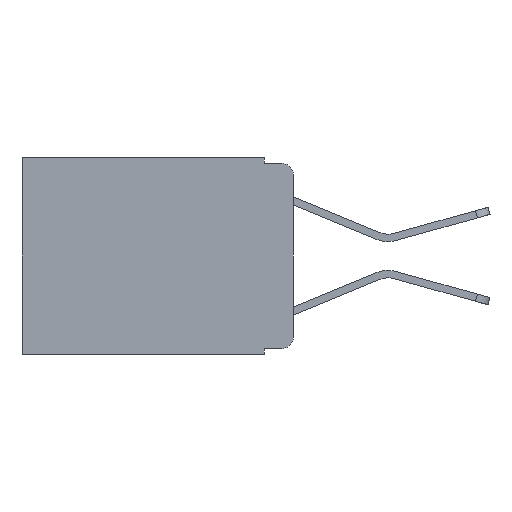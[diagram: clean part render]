
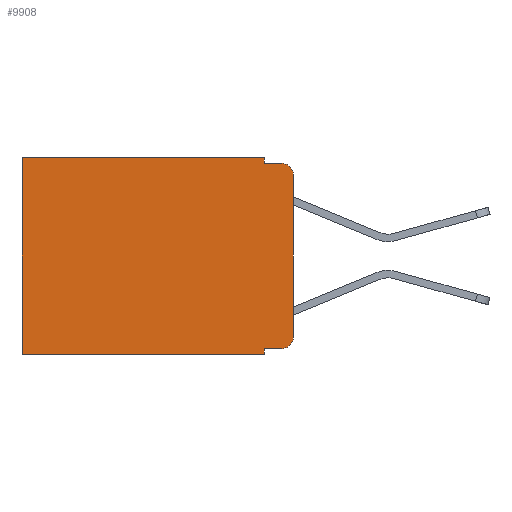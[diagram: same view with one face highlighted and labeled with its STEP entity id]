
A CAD part, left-side view. The second image highlights one B-rep face of the part: STEP entity #9908.
In plain terms, the highlighted planar face has unit normal (-1, 0, 0).
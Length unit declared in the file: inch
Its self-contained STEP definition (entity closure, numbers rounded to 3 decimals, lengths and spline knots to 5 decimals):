
#214 = LINE ( 'NONE', #10549, #2378 ) ;
#764 = ORIENTED_EDGE ( 'NONE', *, *, #7181, .F. ) ;
#981 = ORIENTED_EDGE ( 'NONE', *, *, #8253, .T. ) ;
#994 = ORIENTED_EDGE ( 'NONE', *, *, #7713, .F. ) ;
#1127 = LINE ( 'NONE', #5479, #7815 ) ;
#1152 = DIRECTION ( 'NONE',  ( 1., 0., 0. ) ) ;
#1216 = VECTOR ( 'NONE', #4176, 39.37008 ) ;
#1220 = LINE ( 'NONE', #7101, #10017 ) ;
#1238 = ORIENTED_EDGE ( 'NONE', *, *, #6210, .F. ) ;
#1242 = ORIENTED_EDGE ( 'NONE', *, *, #3553, .F. ) ;
#1414 = ORIENTED_EDGE ( 'NONE', *, *, #7021, .T. ) ;
#1642 = ORIENTED_EDGE ( 'NONE', *, *, #5609, .T. ) ;
#1786 = DIRECTION ( 'NONE',  ( 0., 1., 0. ) ) ;
#1809 = CARTESIAN_POINT ( 'NONE',  ( 0.298, 0.051, -0.01 ) ) ;
#1814 = ORIENTED_EDGE ( 'NONE', *, *, #4394, .T. ) ;
#2066 = DIRECTION ( 'NONE',  ( -1., 0., 0. ) ) ;
#2099 = ORIENTED_EDGE ( 'NONE', *, *, #6758, .T. ) ;
#2120 = CARTESIAN_POINT ( 'NONE',  ( 0.298, 0.02, -0.313 ) ) ;
#2212 = DIRECTION ( 'NONE',  ( 0., 1., 0. ) ) ;
#2268 = ORIENTED_EDGE ( 'NONE', *, *, #2658, .F. ) ;
#2378 = VECTOR ( 'NONE', #2212, 39.37008 ) ;
#2413 = CARTESIAN_POINT ( 'NONE',  ( 0.298, 0., 0. ) ) ;
#2505 = AXIS2_PLACEMENT_3D ( 'NONE', #2120, #9318, #7518 ) ;
#2546 = LINE ( 'NONE', #9538, #7183 ) ;
#2658 = EDGE_CURVE ( 'NONE', #5961, #5140, #1127, .T. ) ;
#2748 = FACE_OUTER_BOUND ( 'NONE', #7191, .T. ) ;
#3095 = CIRCLE ( 'NONE', #2505, 0.02 ) ;
#3159 = DIRECTION ( 'NONE',  ( 0., -1., 0. ) ) ;
#3375 = LINE ( 'NONE', #2413, #1216 ) ;
#3553 = EDGE_CURVE ( 'NONE', #5140, #5456, #2546, .T. ) ;
#4016 = CARTESIAN_POINT ( 'NONE',  ( 0.298, 0.051, -0.01 ) ) ;
#4176 = DIRECTION ( 'NONE',  ( 0., 0., -1. ) ) ;
#4394 = EDGE_CURVE ( 'NONE', #5961, #10137, #1220, .T. ) ;
#4582 = CARTESIAN_POINT ( 'NONE',  ( 0.298, 0.02, -0.01 ) ) ;
#4684 = VECTOR ( 'NONE', #5837, 39.37008 ) ;
#4763 = VERTEX_POINT ( 'NONE', #8011 ) ;
#4827 = CARTESIAN_POINT ( 'NONE',  ( 0.298, 0.051, 0. ) ) ;
#4924 = VERTEX_POINT ( 'NONE', #4582 ) ;
#5134 = LINE ( 'NONE', #4016, #7397 ) ;
#5140 = VERTEX_POINT ( 'NONE', #10711 ) ;
#5454 = DIRECTION ( 'NONE',  ( 0., 0., -1. ) ) ;
#5456 = VERTEX_POINT ( 'NONE', #10879 ) ;
#5479 = CARTESIAN_POINT ( 'NONE',  ( 0.298, 0.051, 0. ) ) ;
#5492 = VERTEX_POINT ( 'NONE', #10755 ) ;
#5609 = EDGE_CURVE ( 'NONE', #9261, #5456, #8527, .T. ) ;
#5837 = DIRECTION ( 'NONE',  ( 0., 0., -1. ) ) ;
#5961 = VERTEX_POINT ( 'NONE', #8649 ) ;
#6088 = VECTOR ( 'NONE', #9145, 39.37008 ) ;
#6210 = EDGE_CURVE ( 'NONE', #4763, #9373, #7249, .T. ) ;
#6714 = AXIS2_PLACEMENT_3D ( 'NONE', #7296, #2066, #8105 ) ;
#6758 = EDGE_CURVE ( 'NONE', #10137, #5492, #3095, .T. ) ;
#6839 = CARTESIAN_POINT ( 'NONE',  ( 0.298, 0.02, -0.333 ) ) ;
#7021 = EDGE_CURVE ( 'NONE', #4763, #9261, #214, .T. ) ;
#7101 = CARTESIAN_POINT ( 'NONE',  ( 0.298, 0.051, -0.333 ) ) ;
#7181 = EDGE_CURVE ( 'NONE', #7731, #5492, #3375, .T. ) ;
#7183 = VECTOR ( 'NONE', #1786, 39.37008 ) ;
#7191 = EDGE_LOOP ( 'NONE', ( #764, #981, #994, #1238, #1414, #1642, #1242, #2268, #1814, #2099 ) ) ;
#7249 = LINE ( 'NONE', #4827, #4684 ) ;
#7275 = CARTESIAN_POINT ( 'NONE',  ( 0.298, 0., 0. ) ) ;
#7296 = CARTESIAN_POINT ( 'NONE',  ( 0.298, 0.02, -0.03 ) ) ;
#7307 = DIRECTION ( 'NONE',  ( 0., 0., -1. ) ) ;
#7397 = VECTOR ( 'NONE', #9065, 39.37008 ) ;
#7518 = DIRECTION ( 'NONE',  ( 0., 0., -1. ) ) ;
#7713 = EDGE_CURVE ( 'NONE', #9373, #4924, #5134, .T. ) ;
#7731 = VERTEX_POINT ( 'NONE', #8292 ) ;
#7815 = VECTOR ( 'NONE', #5454, 39.37008 ) ;
#8011 = CARTESIAN_POINT ( 'NONE',  ( 0.298, 0.051, 0. ) ) ;
#8105 = DIRECTION ( 'NONE',  ( 0., 0., -1. ) ) ;
#8253 = EDGE_CURVE ( 'NONE', #7731, #4924, #9887, .T. ) ;
#8292 = CARTESIAN_POINT ( 'NONE',  ( 0.298, 0., -0.03 ) ) ;
#8527 = LINE ( 'NONE', #8946, #6088 ) ;
#8649 = CARTESIAN_POINT ( 'NONE',  ( 0.298, 0.051, -0.333 ) ) ;
#8737 = AXIS2_PLACEMENT_3D ( 'NONE', #7275, #1152, #7307 ) ;
#8946 = CARTESIAN_POINT ( 'NONE',  ( 0.298, 0.473, 0. ) ) ;
#9065 = DIRECTION ( 'NONE',  ( 0., -1., 0. ) ) ;
#9145 = DIRECTION ( 'NONE',  ( 0., 0., -1. ) ) ;
#9261 = VERTEX_POINT ( 'NONE', #9311 ) ;
#9311 = CARTESIAN_POINT ( 'NONE',  ( 0.298, 0.473, 0. ) ) ;
#9318 = DIRECTION ( 'NONE',  ( -1., 0., 0. ) ) ;
#9373 = VERTEX_POINT ( 'NONE', #1809 ) ;
#9538 = CARTESIAN_POINT ( 'NONE',  ( 0.298, 0., -0.343 ) ) ;
#9676 = PLANE ( 'NONE',  #8737 ) ;
#9887 = CIRCLE ( 'NONE', #6714, 0.02 ) ;
#9908 = ADVANCED_FACE ( 'NONE', ( #2748 ), #9676, .F. ) ;
#10017 = VECTOR ( 'NONE', #3159, 39.37008 ) ;
#10137 = VERTEX_POINT ( 'NONE', #6839 ) ;
#10549 = CARTESIAN_POINT ( 'NONE',  ( 0.298, 0., 0. ) ) ;
#10711 = CARTESIAN_POINT ( 'NONE',  ( 0.298, 0.051, -0.343 ) ) ;
#10755 = CARTESIAN_POINT ( 'NONE',  ( 0.298, 0., -0.313 ) ) ;
#10879 = CARTESIAN_POINT ( 'NONE',  ( 0.298, 0.473, -0.343 ) ) ;
